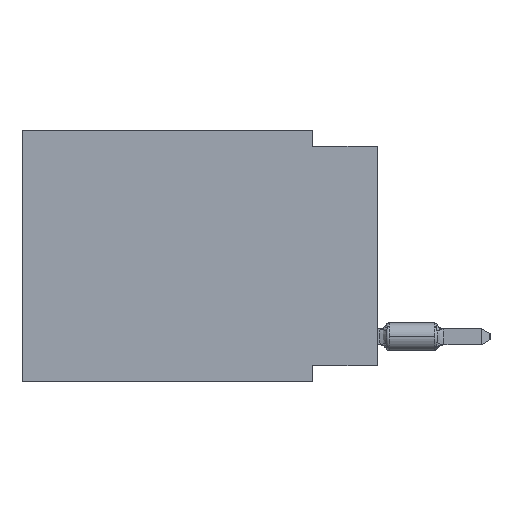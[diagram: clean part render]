
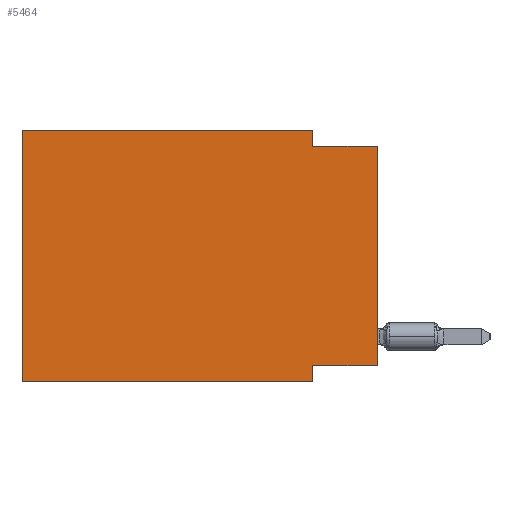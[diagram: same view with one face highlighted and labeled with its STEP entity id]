
A CAD part, left-side view. The second image highlights one B-rep face of the part: STEP entity #5464.
In plain terms, the highlighted planar face has unit normal (-1, 0, 0).
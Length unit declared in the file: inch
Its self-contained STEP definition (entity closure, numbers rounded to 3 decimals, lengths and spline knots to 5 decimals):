
#105 = CARTESIAN_POINT ( 'NONE',  ( 0., 0., -0.025 ) ) ;
#288 = VECTOR ( 'NONE', #5696, 39.37008 ) ;
#674 = LINE ( 'NONE', #18309, #16641 ) ;
#782 = EDGE_CURVE ( 'NONE', #814, #20580, #18489, .T. ) ;
#794 = VERTEX_POINT ( 'NONE', #17628 ) ;
#814 = VERTEX_POINT ( 'NONE', #5845 ) ;
#846 = DIRECTION ( 'NONE',  ( 0., 1., 0. ) ) ;
#1550 = DIRECTION ( 'NONE',  ( 0., 0., 1. ) ) ;
#2048 = LINE ( 'NONE', #13516, #13045 ) ;
#3321 = ORIENTED_EDGE ( 'NONE', *, *, #782, .F. ) ;
#3441 = CARTESIAN_POINT ( 'NONE',  ( 0., 0., -0.025 ) ) ;
#3799 = LINE ( 'NONE', #7288, #288 ) ;
#3832 = VECTOR ( 'NONE', #6274, 39.37008 ) ;
#4005 = CARTESIAN_POINT ( 'NONE',  ( 0., 0.1, -0.365 ) ) ;
#4217 = CARTESIAN_POINT ( 'NONE',  ( 0., 0., 0. ) ) ;
#4836 = CARTESIAN_POINT ( 'NONE',  ( 0., 0.55, 0. ) ) ;
#5464 = ADVANCED_FACE ( 'NONE', ( #16023 ), #12635, .F. ) ;
#5633 = VECTOR ( 'NONE', #6531, 39.37008 ) ;
#5696 = DIRECTION ( 'NONE',  ( 0., 0., -1. ) ) ;
#5729 = VERTEX_POINT ( 'NONE', #10579 ) ;
#5845 = CARTESIAN_POINT ( 'NONE',  ( 0., 0., -0.365 ) ) ;
#6018 = EDGE_CURVE ( 'NONE', #8349, #794, #2048, .T. ) ;
#6033 = DIRECTION ( 'NONE',  ( 0., 0., -1. ) ) ;
#6274 = DIRECTION ( 'NONE',  ( 0., 0., -1. ) ) ;
#6353 = CARTESIAN_POINT ( 'NONE',  ( 0., 0.55, 0. ) ) ;
#6445 = VERTEX_POINT ( 'NONE', #105 ) ;
#6531 = DIRECTION ( 'NONE',  ( 0., -1., 0. ) ) ;
#7018 = LINE ( 'NONE', #4836, #5633 ) ;
#7288 = CARTESIAN_POINT ( 'NONE',  ( 0., 0.1, -0.39 ) ) ;
#7676 = EDGE_CURVE ( 'NONE', #16623, #11867, #7018, .T. ) ;
#8349 = VERTEX_POINT ( 'NONE', #9754 ) ;
#9402 = VECTOR ( 'NONE', #14905, 39.37008 ) ;
#9754 = CARTESIAN_POINT ( 'NONE',  ( 0., 0.55, -0.39 ) ) ;
#9775 = VECTOR ( 'NONE', #846, 39.37008 ) ;
#10355 = EDGE_CURVE ( 'NONE', #5729, #6445, #14802, .T. ) ;
#10579 = CARTESIAN_POINT ( 'NONE',  ( 0., 0.1, -0.025 ) ) ;
#10926 = EDGE_CURVE ( 'NONE', #11867, #5729, #19340, .T. ) ;
#11156 = CARTESIAN_POINT ( 'NONE',  ( 0., 0.1, 0. ) ) ;
#11326 = AXIS2_PLACEMENT_3D ( 'NONE', #6353, #18898, #6033 ) ;
#11361 = ORIENTED_EDGE ( 'NONE', *, *, #7676, .F. ) ;
#11417 = EDGE_CURVE ( 'NONE', #8349, #16623, #674, .T. ) ;
#11610 = CARTESIAN_POINT ( 'NONE',  ( 0., 0.1, 0. ) ) ;
#11867 = VERTEX_POINT ( 'NONE', #11610 ) ;
#12635 = PLANE ( 'NONE',  #11326 ) ;
#12853 = ORIENTED_EDGE ( 'NONE', *, *, #6018, .T. ) ;
#13045 = VECTOR ( 'NONE', #15008, 39.37008 ) ;
#13238 = ORIENTED_EDGE ( 'NONE', *, *, #10355, .F. ) ;
#13516 = CARTESIAN_POINT ( 'NONE',  ( 0., 0.55, -0.39 ) ) ;
#14802 = LINE ( 'NONE', #3441, #9402 ) ;
#14905 = DIRECTION ( 'NONE',  ( 0., -1., 0. ) ) ;
#15008 = DIRECTION ( 'NONE',  ( 0., -1., 0. ) ) ;
#15414 = CARTESIAN_POINT ( 'NONE',  ( 0., 0., -0.365 ) ) ;
#16023 = FACE_OUTER_BOUND ( 'NONE', #21021, .T. ) ;
#16623 = VERTEX_POINT ( 'NONE', #17996 ) ;
#16641 = VECTOR ( 'NONE', #16923, 39.37008 ) ;
#16923 = DIRECTION ( 'NONE',  ( 0., 0., 1. ) ) ;
#17620 = EDGE_CURVE ( 'NONE', #814, #6445, #18764, .T. ) ;
#17628 = CARTESIAN_POINT ( 'NONE',  ( 0., 0.1, -0.39 ) ) ;
#17996 = CARTESIAN_POINT ( 'NONE',  ( 0., 0.55, 0. ) ) ;
#18126 = VECTOR ( 'NONE', #1550, 39.37008 ) ;
#18209 = ORIENTED_EDGE ( 'NONE', *, *, #19380, .F. ) ;
#18309 = CARTESIAN_POINT ( 'NONE',  ( 0., 0.55, 0. ) ) ;
#18353 = ORIENTED_EDGE ( 'NONE', *, *, #17620, .T. ) ;
#18489 = LINE ( 'NONE', #15414, #9775 ) ;
#18553 = ORIENTED_EDGE ( 'NONE', *, *, #10926, .F. ) ;
#18764 = LINE ( 'NONE', #4217, #18126 ) ;
#18898 = DIRECTION ( 'NONE',  ( 1., 0., 0. ) ) ;
#18909 = ORIENTED_EDGE ( 'NONE', *, *, #11417, .F. ) ;
#19340 = LINE ( 'NONE', #11156, #3832 ) ;
#19380 = EDGE_CURVE ( 'NONE', #20580, #794, #3799, .T. ) ;
#20580 = VERTEX_POINT ( 'NONE', #4005 ) ;
#21021 = EDGE_LOOP ( 'NONE', ( #18353, #13238, #18553, #11361, #18909, #12853, #18209, #3321 ) ) ;
